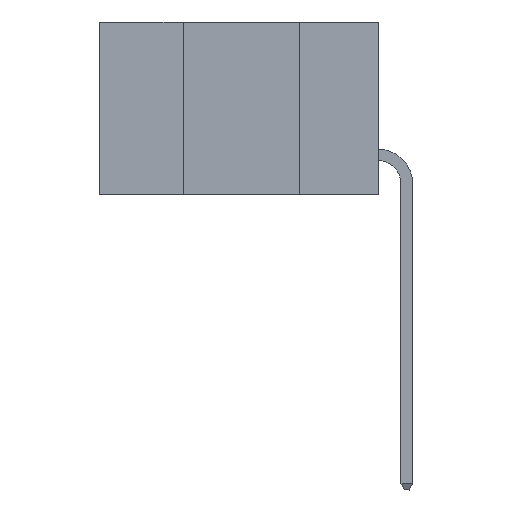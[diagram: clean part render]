
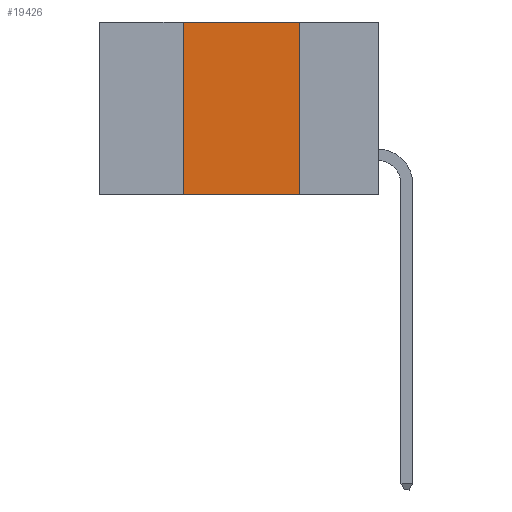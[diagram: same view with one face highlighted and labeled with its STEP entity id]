
A CAD part, left-side view. The second image highlights one B-rep face of the part: STEP entity #19426.
In plain terms, the highlighted planar face has unit normal (-1, 0, 0).
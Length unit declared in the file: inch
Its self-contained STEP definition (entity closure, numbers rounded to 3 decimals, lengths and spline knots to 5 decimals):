
#165 = EDGE_CURVE ( 'NONE', #17037, #22585, #19017, .T. ) ;
#930 = CARTESIAN_POINT ( 'NONE',  ( 0., 0.42, 0. ) ) ;
#1991 = EDGE_CURVE ( 'NONE', #20279, #23193, #12332, .T. ) ;
#2502 = AXIS2_PLACEMENT_3D ( 'NONE', #9551, #17022, #9195 ) ;
#2907 = CARTESIAN_POINT ( 'NONE',  ( 0., 0.42, -0.37 ) ) ;
#3302 = ORIENTED_EDGE ( 'NONE', *, *, #24085, .T. ) ;
#3800 = CARTESIAN_POINT ( 'NONE',  ( 0., 0.17, -0.37 ) ) ;
#3850 = VECTOR ( 'NONE', #20960, 39.37008 ) ;
#5013 = VECTOR ( 'NONE', #23245, 39.37008 ) ;
#5674 = EDGE_LOOP ( 'NONE', ( #23198, #11120, #9651, #3302 ) ) ;
#9195 = DIRECTION ( 'NONE',  ( 0., 0., -1. ) ) ;
#9551 = CARTESIAN_POINT ( 'NONE',  ( 0., 0.6, 0. ) ) ;
#9600 = CARTESIAN_POINT ( 'NONE',  ( 0., 0.17, -0.37 ) ) ;
#9651 = ORIENTED_EDGE ( 'NONE', *, *, #1991, .F. ) ;
#11120 = ORIENTED_EDGE ( 'NONE', *, *, #23479, .F. ) ;
#12332 = LINE ( 'NONE', #17912, #5013 ) ;
#12544 = VECTOR ( 'NONE', #19404, 39.37008 ) ;
#14216 = CARTESIAN_POINT ( 'NONE',  ( 0., 0.17, 0. ) ) ;
#15090 = PLANE ( 'NONE',  #2502 ) ;
#17022 = DIRECTION ( 'NONE',  ( 1., 0., 0. ) ) ;
#17037 = VERTEX_POINT ( 'NONE', #14216 ) ;
#17136 = LINE ( 'NONE', #19097, #3850 ) ;
#17717 = DIRECTION ( 'NONE',  ( 0., -1., 0. ) ) ;
#17912 = CARTESIAN_POINT ( 'NONE',  ( 0., 0.42, -0.37 ) ) ;
#18618 = FACE_OUTER_BOUND ( 'NONE', #5674, .T. ) ;
#19017 = LINE ( 'NONE', #9600, #12544 ) ;
#19097 = CARTESIAN_POINT ( 'NONE',  ( 0., 0.6, 0. ) ) ;
#19404 = DIRECTION ( 'NONE',  ( 0., 0., -1. ) ) ;
#19426 = ADVANCED_FACE ( 'NONE', ( #18618 ), #15090, .F. ) ;
#19518 = VECTOR ( 'NONE', #17717, 39.37008 ) ;
#20279 = VERTEX_POINT ( 'NONE', #2907 ) ;
#20960 = DIRECTION ( 'NONE',  ( 0., -1., 0. ) ) ;
#21294 = LINE ( 'NONE', #21417, #19518 ) ;
#21417 = CARTESIAN_POINT ( 'NONE',  ( 0., 0.6, -0.37 ) ) ;
#22585 = VERTEX_POINT ( 'NONE', #3800 ) ;
#23193 = VERTEX_POINT ( 'NONE', #930 ) ;
#23198 = ORIENTED_EDGE ( 'NONE', *, *, #165, .F. ) ;
#23245 = DIRECTION ( 'NONE',  ( 0., 0., 1. ) ) ;
#23479 = EDGE_CURVE ( 'NONE', #23193, #17037, #17136, .T. ) ;
#24085 = EDGE_CURVE ( 'NONE', #20279, #22585, #21294, .T. ) ;
